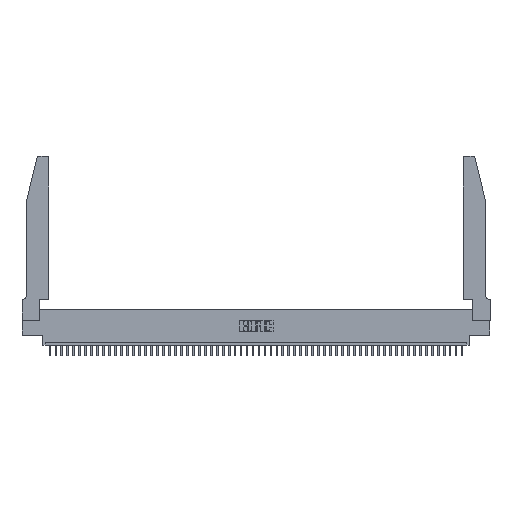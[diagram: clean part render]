
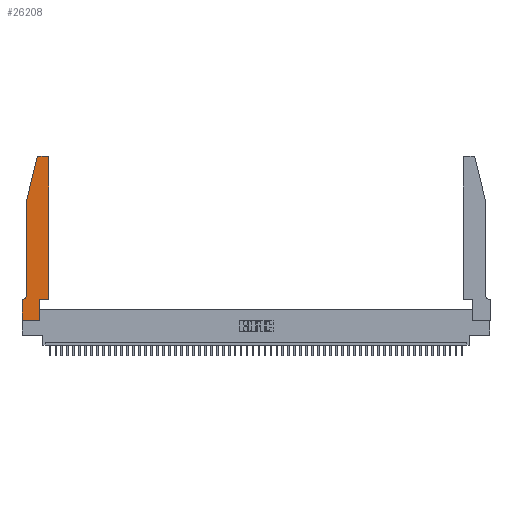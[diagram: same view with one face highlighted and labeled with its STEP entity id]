
A CAD part, top view. The second image highlights one B-rep face of the part: STEP entity #26208.
In plain terms, the highlighted planar face has unit normal (0, 0, 1).
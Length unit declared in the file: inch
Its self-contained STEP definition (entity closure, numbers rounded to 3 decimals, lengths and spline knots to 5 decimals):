
#1477 = DIRECTION ( 'NONE',  ( 0., 0., 1. ) ) ;
#1984 = EDGE_CURVE ( 'NONE', #11942, #23193, #27926, .T. ) ;
#2683 = CARTESIAN_POINT ( 'NONE',  ( 0.0055, 0.42, 0.37 ) ) ;
#3259 = CARTESIAN_POINT ( 'NONE',  ( 0.2605, 2.75, 0.37 ) ) ;
#3376 = CARTESIAN_POINT ( 'NONE',  ( 0.0755, 2., 0.37 ) ) ;
#5525 = PLANE ( 'NONE',  #49873 ) ;
#5884 = LINE ( 'NONE', #21479, #11189 ) ;
#6661 = CARTESIAN_POINT ( 'NONE',  ( 0., 0., 0.37 ) ) ;
#7090 = VECTOR ( 'NONE', #16773, 39.37008 ) ;
#7890 = CARTESIAN_POINT ( 'NONE',  ( 0.2865, 0.35, 0.37 ) ) ;
#7997 = VERTEX_POINT ( 'NONE', #35340 ) ;
#10156 = CARTESIAN_POINT ( 'NONE',  ( 0.0755, 0.35, 0.37 ) ) ;
#10484 = CARTESIAN_POINT ( 'NONE',  ( 0., 0.35, 0.37 ) ) ;
#10851 = VERTEX_POINT ( 'NONE', #52724 ) ;
#11081 = DIRECTION ( 'NONE',  ( -1., 0., 0. ) ) ;
#11189 = VECTOR ( 'NONE', #25484, 39.37008 ) ;
#11621 = CARTESIAN_POINT ( 'NONE',  ( 0.4205, 2.72, 0.37 ) ) ;
#11942 = VERTEX_POINT ( 'NONE', #51223 ) ;
#13468 = VECTOR ( 'NONE', #32573, 39.37008 ) ;
#13529 = CARTESIAN_POINT ( 'NONE',  ( 0.2865, 0.35, 0.37 ) ) ;
#14203 = EDGE_CURVE ( 'NONE', #49131, #43462, #27282, .T. ) ;
#14284 = VECTOR ( 'NONE', #43667, 39.37008 ) ;
#14691 = FACE_OUTER_BOUND ( 'NONE', #50069, .T. ) ;
#14991 = EDGE_CURVE ( 'NONE', #44608, #49131, #28555, .T. ) ;
#15308 = AXIS2_PLACEMENT_3D ( 'NONE', #11621, #33277, #49497 ) ;
#15963 = EDGE_CURVE ( 'NONE', #28865, #7997, #36932, .T. ) ;
#16773 = DIRECTION ( 'NONE',  ( 0., 1., 0. ) ) ;
#17310 = VECTOR ( 'NONE', #42417, 39.37008 ) ;
#17904 = LINE ( 'NONE', #42593, #17310 ) ;
#20533 = ORIENTED_EDGE ( 'NONE', *, *, #45053, .T. ) ;
#21479 = CARTESIAN_POINT ( 'NONE',  ( 0.4505, 0.35, 0.37 ) ) ;
#22012 = DIRECTION ( 'NONE',  ( 0., 0., 1. ) ) ;
#22349 = CARTESIAN_POINT ( 'NONE',  ( 0.4505, 0.35, 0.37 ) ) ;
#22800 = DIRECTION ( 'NONE',  ( 0., -1., 0. ) ) ;
#23179 = VECTOR ( 'NONE', #26470, 39.37008 ) ;
#23193 = VERTEX_POINT ( 'NONE', #13529 ) ;
#23832 = DIRECTION ( 'NONE',  ( -1., 0., 0. ) ) ;
#23918 = CARTESIAN_POINT ( 'NONE',  ( 0., 0., 0.37 ) ) ;
#24641 = EDGE_CURVE ( 'NONE', #25172, #10851, #51182, .T. ) ;
#24732 = EDGE_CURVE ( 'NONE', #10851, #44608, #17904, .T. ) ;
#25172 = VERTEX_POINT ( 'NONE', #37774 ) ;
#25484 = DIRECTION ( 'NONE',  ( 1., 0., 0. ) ) ;
#26208 = ADVANCED_FACE ( 'NONE', ( #14691 ), #5525, .T. ) ;
#26393 = CARTESIAN_POINT ( 'NONE',  ( 0.4505, 2.72, 0.37 ) ) ;
#26470 = DIRECTION ( 'NONE',  ( 1., 0., 0. ) ) ;
#26656 = CARTESIAN_POINT ( 'NONE',  ( 0., 0., 0.37 ) ) ;
#26965 = ORIENTED_EDGE ( 'NONE', *, *, #1984, .T. ) ;
#27282 = CIRCLE ( 'NONE', #40772, 0.07 ) ;
#27926 = LINE ( 'NONE', #7890, #7090 ) ;
#28430 = LINE ( 'NONE', #3259, #44726 ) ;
#28555 = LINE ( 'NONE', #3376, #13468 ) ;
#28865 = VERTEX_POINT ( 'NONE', #26393 ) ;
#29839 = VECTOR ( 'NONE', #46914, 39.37008 ) ;
#30063 = EDGE_CURVE ( 'NONE', #46108, #28865, #51385, .T. ) ;
#30586 = DIRECTION ( 'NONE',  ( 1., 0., 0. ) ) ;
#30668 = DIRECTION ( 'NONE',  ( 1., 0., 0. ) ) ;
#31808 = ORIENTED_EDGE ( 'NONE', *, *, #52118, .T. ) ;
#31874 = DIRECTION ( 'NONE',  ( 0., 0., -1. ) ) ;
#31883 = EDGE_CURVE ( 'NONE', #34506, #11942, #33656, .T. ) ;
#32573 = DIRECTION ( 'NONE',  ( 0., -1., 0. ) ) ;
#32586 = ORIENTED_EDGE ( 'NONE', *, *, #46387, .T. ) ;
#32816 = ORIENTED_EDGE ( 'NONE', *, *, #24732, .T. ) ;
#33277 = DIRECTION ( 'NONE',  ( 0., 0., 1. ) ) ;
#33656 = LINE ( 'NONE', #26656, #23179 ) ;
#33798 = VECTOR ( 'NONE', #22800, 39.37008 ) ;
#34506 = VERTEX_POINT ( 'NONE', #23918 ) ;
#34771 = CARTESIAN_POINT ( 'NONE',  ( 0.284, 2.72, 0.37 ) ) ;
#35340 = CARTESIAN_POINT ( 'NONE',  ( 0.4205, 2.75, 0.37 ) ) ;
#35383 = ORIENTED_EDGE ( 'NONE', *, *, #24641, .T. ) ;
#35821 = ORIENTED_EDGE ( 'NONE', *, *, #30063, .T. ) ;
#36932 = CIRCLE ( 'NONE', #15308, 0.03 ) ;
#37315 = ORIENTED_EDGE ( 'NONE', *, *, #31883, .T. ) ;
#37774 = CARTESIAN_POINT ( 'NONE',  ( 0.284, 2.75, 0.37 ) ) ;
#39262 = CARTESIAN_POINT ( 'NONE',  ( 0.0055, 0.35, 0.37 ) ) ;
#39766 = CARTESIAN_POINT ( 'NONE',  ( 0.0755, 0.42, 0.37 ) ) ;
#40772 = AXIS2_PLACEMENT_3D ( 'NONE', #2683, #31874, #11081 ) ;
#41128 = ORIENTED_EDGE ( 'NONE', *, *, #15963, .T. ) ;
#41159 = ORIENTED_EDGE ( 'NONE', *, *, #50234, .T. ) ;
#42417 = DIRECTION ( 'NONE',  ( -0.239, -0.971, 0. ) ) ;
#42593 = CARTESIAN_POINT ( 'NONE',  ( 0.0755, 2., 0.37 ) ) ;
#43462 = VERTEX_POINT ( 'NONE', #39262 ) ;
#43667 = DIRECTION ( 'NONE',  ( 0., 1., 0. ) ) ;
#44012 = ORIENTED_EDGE ( 'NONE', *, *, #14991, .T. ) ;
#44608 = VERTEX_POINT ( 'NONE', #52582 ) ;
#44726 = VECTOR ( 'NONE', #23832, 39.37008 ) ;
#45053 = EDGE_CURVE ( 'NONE', #46192, #34506, #48133, .T. ) ;
#46108 = VERTEX_POINT ( 'NONE', #50708 ) ;
#46192 = VERTEX_POINT ( 'NONE', #10484 ) ;
#46387 = EDGE_CURVE ( 'NONE', #7997, #25172, #28430, .T. ) ;
#46914 = DIRECTION ( 'NONE',  ( -1., 0., 0. ) ) ;
#47235 = CARTESIAN_POINT ( 'NONE',  ( 0., 0.35, 0.37 ) ) ;
#48127 = LINE ( 'NONE', #10156, #29839 ) ;
#48133 = LINE ( 'NONE', #6661, #33798 ) ;
#49067 = AXIS2_PLACEMENT_3D ( 'NONE', #34771, #22012, #30586 ) ;
#49131 = VERTEX_POINT ( 'NONE', #39766 ) ;
#49497 = DIRECTION ( 'NONE',  ( 1., 0., 0. ) ) ;
#49873 = AXIS2_PLACEMENT_3D ( 'NONE', #47235, #1477, #30668 ) ;
#50069 = EDGE_LOOP ( 'NONE', ( #32586, #35383, #32816, #44012, #52355, #31808, #20533, #37315, #26965, #41159, #35821, #41128 ) ) ;
#50234 = EDGE_CURVE ( 'NONE', #23193, #46108, #5884, .T. ) ;
#50708 = CARTESIAN_POINT ( 'NONE',  ( 0.4505, 0.35, 0.37 ) ) ;
#51182 = CIRCLE ( 'NONE', #49067, 0.03 ) ;
#51223 = CARTESIAN_POINT ( 'NONE',  ( 0.2865, 0., 0.37 ) ) ;
#51385 = LINE ( 'NONE', #22349, #14284 ) ;
#52118 = EDGE_CURVE ( 'NONE', #43462, #46192, #48127, .T. ) ;
#52355 = ORIENTED_EDGE ( 'NONE', *, *, #14203, .T. ) ;
#52582 = CARTESIAN_POINT ( 'NONE',  ( 0.0755, 2., 0.37 ) ) ;
#52724 = CARTESIAN_POINT ( 'NONE',  ( 0.25487, 2.72718, 0.37 ) ) ;
